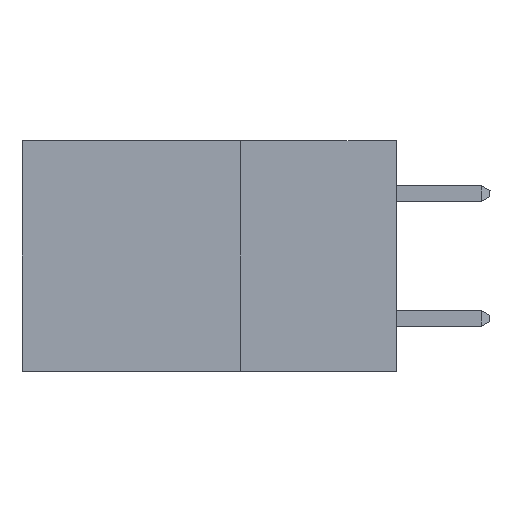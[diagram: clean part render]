
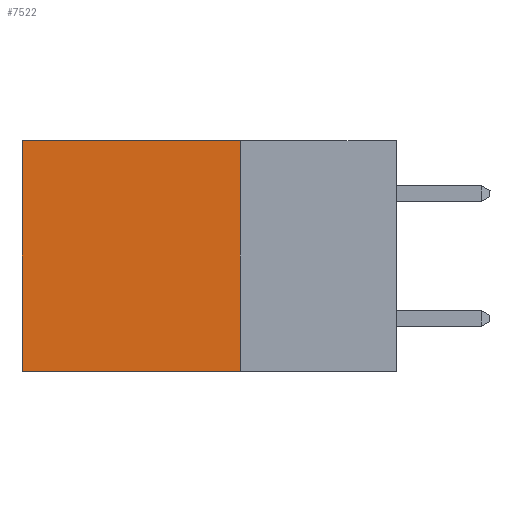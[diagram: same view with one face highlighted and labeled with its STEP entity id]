
A CAD part, left-side view. The second image highlights one B-rep face of the part: STEP entity #7522.
In plain terms, the highlighted planar face has unit normal (-1, 0, 0).
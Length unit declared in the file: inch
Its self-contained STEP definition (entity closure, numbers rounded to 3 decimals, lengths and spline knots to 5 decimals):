
#37 = CARTESIAN_POINT ( 'NONE',  ( 0.298, 0.6, 0. ) ) ;
#493 = EDGE_CURVE ( 'NONE', #20424, #5992, #21458, .T. ) ;
#1035 = CARTESIAN_POINT ( 'NONE',  ( 0.298, 0.6, 0. ) ) ;
#2701 = ORIENTED_EDGE ( 'NONE', *, *, #13190, .F. ) ;
#3196 = CARTESIAN_POINT ( 'NONE',  ( 0.298, 0.25, 0. ) ) ;
#5050 = VERTEX_POINT ( 'NONE', #37 ) ;
#5132 = DIRECTION ( 'NONE',  ( 0., 0., -1. ) ) ;
#5689 = ORIENTED_EDGE ( 'NONE', *, *, #10952, .T. ) ;
#5874 = FACE_OUTER_BOUND ( 'NONE', #8636, .T. ) ;
#5992 = VERTEX_POINT ( 'NONE', #10316 ) ;
#7327 = VERTEX_POINT ( 'NONE', #16039 ) ;
#7494 = AXIS2_PLACEMENT_3D ( 'NONE', #3196, #16599, #5132 ) ;
#7522 = ADVANCED_FACE ( 'NONE', ( #5874 ), #14708, .F. ) ;
#8445 = LINE ( 'NONE', #1035, #23056 ) ;
#8636 = EDGE_LOOP ( 'NONE', ( #5689, #2701, #16247, #12841 ) ) ;
#9520 = VECTOR ( 'NONE', #12872, 39.37008 ) ;
#10316 = CARTESIAN_POINT ( 'NONE',  ( 0.298, 0.25, -0.37 ) ) ;
#10952 = EDGE_CURVE ( 'NONE', #5050, #7327, #8445, .T. ) ;
#11135 = DIRECTION ( 'NONE',  ( 0., 0., -1. ) ) ;
#11513 = CARTESIAN_POINT ( 'NONE',  ( 0.298, 0.25, -0.37 ) ) ;
#12841 = ORIENTED_EDGE ( 'NONE', *, *, #19352, .T. ) ;
#12872 = DIRECTION ( 'NONE',  ( 0., 1., 0. ) ) ;
#13190 = EDGE_CURVE ( 'NONE', #5992, #7327, #14644, .T. ) ;
#14046 = VECTOR ( 'NONE', #15345, 39.37008 ) ;
#14644 = LINE ( 'NONE', #11513, #14046 ) ;
#14708 = PLANE ( 'NONE',  #7494 ) ;
#15345 = DIRECTION ( 'NONE',  ( 0., 1., 0. ) ) ;
#15816 = VECTOR ( 'NONE', #11135, 39.37008 ) ;
#16039 = CARTESIAN_POINT ( 'NONE',  ( 0.298, 0.6, -0.37 ) ) ;
#16247 = ORIENTED_EDGE ( 'NONE', *, *, #493, .F. ) ;
#16599 = DIRECTION ( 'NONE',  ( 1., 0., 0. ) ) ;
#19352 = EDGE_CURVE ( 'NONE', #20424, #5050, #24141, .T. ) ;
#20424 = VERTEX_POINT ( 'NONE', #21449 ) ;
#21057 = CARTESIAN_POINT ( 'NONE',  ( 0.298, 0.25, 0. ) ) ;
#21449 = CARTESIAN_POINT ( 'NONE',  ( 0.298, 0.25, 0. ) ) ;
#21458 = LINE ( 'NONE', #21057, #15816 ) ;
#23056 = VECTOR ( 'NONE', #23993, 39.37008 ) ;
#23993 = DIRECTION ( 'NONE',  ( 0., 0., -1. ) ) ;
#24141 = LINE ( 'NONE', #24239, #9520 ) ;
#24239 = CARTESIAN_POINT ( 'NONE',  ( 0.298, 0.25, 0. ) ) ;
